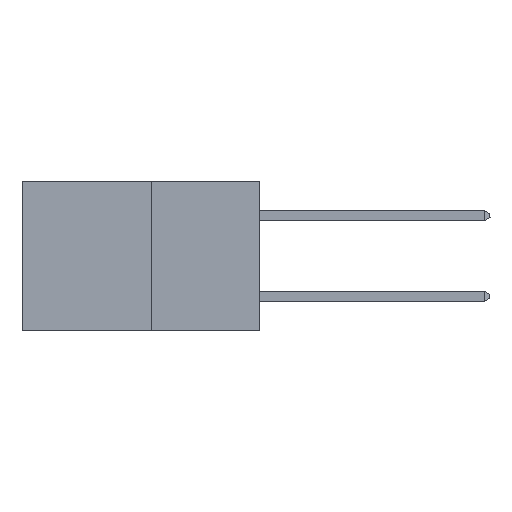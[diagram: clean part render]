
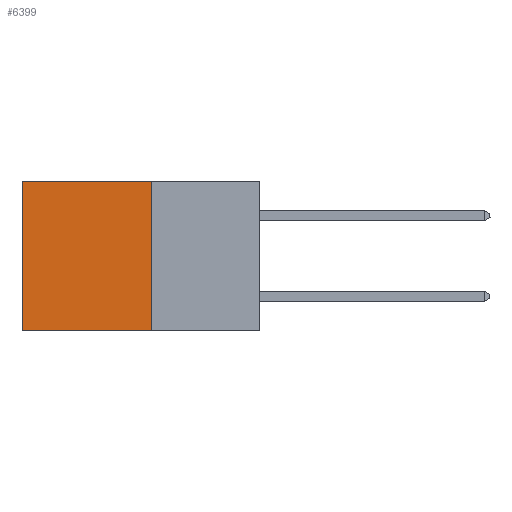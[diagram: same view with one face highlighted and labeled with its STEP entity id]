
A CAD part, left-side view. The second image highlights one B-rep face of the part: STEP entity #6399.
In plain terms, the highlighted planar face has unit normal (-1, 0, 0).
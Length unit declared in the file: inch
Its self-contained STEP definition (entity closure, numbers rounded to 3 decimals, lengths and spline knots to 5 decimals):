
#499 = EDGE_CURVE ( 'NONE', #18562, #17392, #14157, .T. ) ;
#1682 = LINE ( 'NONE', #12154, #13588 ) ;
#2368 = CARTESIAN_POINT ( 'NONE',  ( 0.277, 0.59, -0.37 ) ) ;
#3014 = DIRECTION ( 'NONE',  ( 0., 0., -1. ) ) ;
#3682 = DIRECTION ( 'NONE',  ( 0., 0., -1. ) ) ;
#4159 = VECTOR ( 'NONE', #11745, 39.37008 ) ;
#5435 = ORIENTED_EDGE ( 'NONE', *, *, #7942, .T. ) ;
#6045 = VECTOR ( 'NONE', #3014, 39.37008 ) ;
#6399 = ADVANCED_FACE ( 'NONE', ( #11353 ), #17281, .F. ) ;
#6753 = ORIENTED_EDGE ( 'NONE', *, *, #499, .F. ) ;
#6800 = AXIS2_PLACEMENT_3D ( 'NONE', #9913, #12972, #3682 ) ;
#7851 = CARTESIAN_POINT ( 'NONE',  ( 0.277, 0.27, -0.37 ) ) ;
#7890 = CARTESIAN_POINT ( 'NONE',  ( 0.277, 0.59, -0.37 ) ) ;
#7942 = EDGE_CURVE ( 'NONE', #17023, #17392, #8825, .T. ) ;
#8111 = VERTEX_POINT ( 'NONE', #14992 ) ;
#8825 = LINE ( 'NONE', #2368, #4159 ) ;
#8960 = ORIENTED_EDGE ( 'NONE', *, *, #15238, .F. ) ;
#9913 = CARTESIAN_POINT ( 'NONE',  ( 0.277, 0.27, -0.37 ) ) ;
#10187 = VECTOR ( 'NONE', #11044, 39.37008 ) ;
#10196 = EDGE_LOOP ( 'NONE', ( #5435, #6753, #8960, #19237 ) ) ;
#11044 = DIRECTION ( 'NONE',  ( 0., 1., 0. ) ) ;
#11198 = LINE ( 'NONE', #15257, #6045 ) ;
#11353 = FACE_OUTER_BOUND ( 'NONE', #10196, .T. ) ;
#11745 = DIRECTION ( 'NONE',  ( 0., 0., -1. ) ) ;
#11755 = EDGE_CURVE ( 'NONE', #8111, #17023, #1682, .T. ) ;
#12154 = CARTESIAN_POINT ( 'NONE',  ( 0.277, 0.27, 0. ) ) ;
#12972 = DIRECTION ( 'NONE',  ( 1., 0., 0. ) ) ;
#13588 = VECTOR ( 'NONE', #14997, 39.37008 ) ;
#14157 = LINE ( 'NONE', #15490, #10187 ) ;
#14992 = CARTESIAN_POINT ( 'NONE',  ( 0.277, 0.27, 0. ) ) ;
#14997 = DIRECTION ( 'NONE',  ( 0., 1., 0. ) ) ;
#15238 = EDGE_CURVE ( 'NONE', #8111, #18562, #11198, .T. ) ;
#15257 = CARTESIAN_POINT ( 'NONE',  ( 0.277, 0.27, -0.37 ) ) ;
#15490 = CARTESIAN_POINT ( 'NONE',  ( 0.277, 0.27, -0.37 ) ) ;
#17023 = VERTEX_POINT ( 'NONE', #19067 ) ;
#17281 = PLANE ( 'NONE',  #6800 ) ;
#17392 = VERTEX_POINT ( 'NONE', #7890 ) ;
#18562 = VERTEX_POINT ( 'NONE', #7851 ) ;
#19067 = CARTESIAN_POINT ( 'NONE',  ( 0.277, 0.59, 0. ) ) ;
#19237 = ORIENTED_EDGE ( 'NONE', *, *, #11755, .T. ) ;
